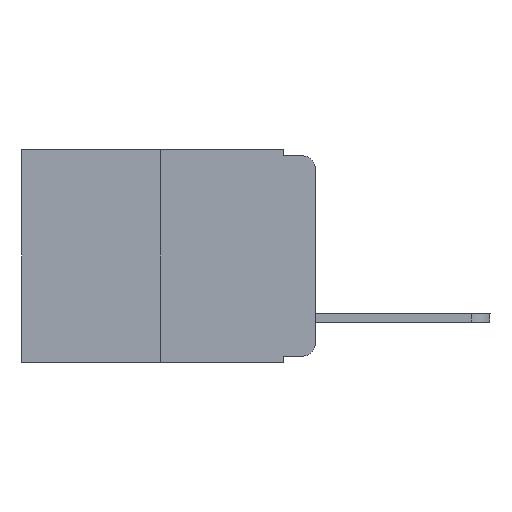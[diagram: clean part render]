
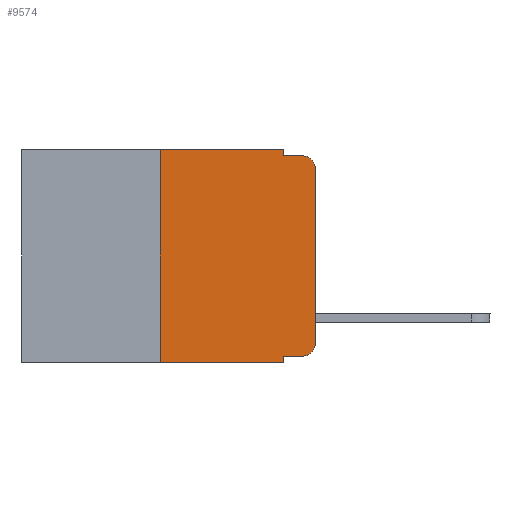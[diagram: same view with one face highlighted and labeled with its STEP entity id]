
A CAD part, left-side view. The second image highlights one B-rep face of the part: STEP entity #9574.
In plain terms, the highlighted planar face has unit normal (-1, 0, 0).
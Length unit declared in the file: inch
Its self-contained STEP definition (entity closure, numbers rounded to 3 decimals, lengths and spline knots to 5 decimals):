
#518 = CARTESIAN_POINT ( 'NONE',  ( 0., 0.02, -0.03 ) ) ;
#831 = DIRECTION ( 'NONE',  ( -1., 0., 0. ) ) ;
#873 = EDGE_LOOP ( 'NONE', ( #3784, #8087, #7034, #19540, #10809, #8668, #8535, #2222, #12883, #15173 ) ) ;
#1061 = LINE ( 'NONE', #19405, #1389 ) ;
#1174 = CARTESIAN_POINT ( 'NONE',  ( 0., 0.02, -0.313 ) ) ;
#1389 = VECTOR ( 'NONE', #11423, 39.37008 ) ;
#1435 = LINE ( 'NONE', #15601, #15882 ) ;
#1588 = CARTESIAN_POINT ( 'NONE',  ( 0., 0.051, 0. ) ) ;
#1994 = LINE ( 'NONE', #3849, #14591 ) ;
#2222 = ORIENTED_EDGE ( 'NONE', *, *, #19116, .F. ) ;
#2387 = EDGE_CURVE ( 'NONE', #11738, #17434, #1435, .T. ) ;
#3282 = CARTESIAN_POINT ( 'NONE',  ( 0., 0., -0.03 ) ) ;
#3784 = ORIENTED_EDGE ( 'NONE', *, *, #24043, .T. ) ;
#3849 = CARTESIAN_POINT ( 'NONE',  ( 0., 0., 0. ) ) ;
#4148 = AXIS2_PLACEMENT_3D ( 'NONE', #518, #22100, #8493 ) ;
#5404 = CARTESIAN_POINT ( 'NONE',  ( 0., 0.051, -0.333 ) ) ;
#6978 = LINE ( 'NONE', #7891, #9766 ) ;
#7034 = ORIENTED_EDGE ( 'NONE', *, *, #2387, .F. ) ;
#7045 = DIRECTION ( 'NONE',  ( 0., 0., 1. ) ) ;
#7232 = EDGE_CURVE ( 'NONE', #15763, #18073, #17824, .T. ) ;
#7244 = CIRCLE ( 'NONE', #4148, 0.02 ) ;
#7891 = CARTESIAN_POINT ( 'NONE',  ( 0., 0.051, 0. ) ) ;
#8087 = ORIENTED_EDGE ( 'NONE', *, *, #24436, .T. ) ;
#8136 = CARTESIAN_POINT ( 'NONE',  ( 0., 0.02, -0.01 ) ) ;
#8482 = CARTESIAN_POINT ( 'NONE',  ( 0., 0.051, -0.333 ) ) ;
#8493 = DIRECTION ( 'NONE',  ( 0., 0., -1. ) ) ;
#8535 = ORIENTED_EDGE ( 'NONE', *, *, #22345, .T. ) ;
#8668 = ORIENTED_EDGE ( 'NONE', *, *, #12371, .F. ) ;
#9007 = VERTEX_POINT ( 'NONE', #13498 ) ;
#9574 = ADVANCED_FACE ( 'NONE', ( #18085 ), #23467, .F. ) ;
#9766 = VECTOR ( 'NONE', #11750, 39.37008 ) ;
#10382 = DIRECTION ( 'NONE',  ( 0., -1., 0. ) ) ;
#10468 = LINE ( 'NONE', #23230, #25074 ) ;
#10804 = DIRECTION ( 'NONE',  ( 0., 0., -1. ) ) ;
#10809 = ORIENTED_EDGE ( 'NONE', *, *, #19938, .F. ) ;
#10907 = CARTESIAN_POINT ( 'NONE',  ( 0., 0.051, -0.01 ) ) ;
#11133 = EDGE_CURVE ( 'NONE', #13557, #11738, #1061, .T. ) ;
#11423 = DIRECTION ( 'NONE',  ( 0., 0., -1. ) ) ;
#11502 = VERTEX_POINT ( 'NONE', #3282 ) ;
#11738 = VERTEX_POINT ( 'NONE', #10907 ) ;
#11750 = DIRECTION ( 'NONE',  ( 0., 0., -1. ) ) ;
#12371 = EDGE_CURVE ( 'NONE', #20728, #12665, #13616, .T. ) ;
#12623 = VECTOR ( 'NONE', #10382, 39.37008 ) ;
#12665 = VERTEX_POINT ( 'NONE', #19398 ) ;
#12883 = ORIENTED_EDGE ( 'NONE', *, *, #7232, .T. ) ;
#13142 = DIRECTION ( 'NONE',  ( 0., 0., -1. ) ) ;
#13294 = VECTOR ( 'NONE', #22021, 39.37008 ) ;
#13498 = CARTESIAN_POINT ( 'NONE',  ( 0., 0., -0.313 ) ) ;
#13557 = VERTEX_POINT ( 'NONE', #1588 ) ;
#13616 = LINE ( 'NONE', #14292, #13294 ) ;
#13661 = CARTESIAN_POINT ( 'NONE',  ( 0., 0.25, -0.343 ) ) ;
#13800 = DIRECTION ( 'NONE',  ( 0., -1., 0. ) ) ;
#14292 = CARTESIAN_POINT ( 'NONE',  ( 0., 0.25, 0. ) ) ;
#14591 = VECTOR ( 'NONE', #7045, 39.37008 ) ;
#15173 = ORIENTED_EDGE ( 'NONE', *, *, #25037, .T. ) ;
#15601 = CARTESIAN_POINT ( 'NONE',  ( 0., 0.051, -0.01 ) ) ;
#15632 = DIRECTION ( 'NONE',  ( 1., 0., 0. ) ) ;
#15763 = VERTEX_POINT ( 'NONE', #5404 ) ;
#15882 = VECTOR ( 'NONE', #13800, 39.37008 ) ;
#16668 = AXIS2_PLACEMENT_3D ( 'NONE', #1174, #831, #10804 ) ;
#16928 = CARTESIAN_POINT ( 'NONE',  ( 0., 0.051, -0.343 ) ) ;
#17381 = LINE ( 'NONE', #24746, #21279 ) ;
#17434 = VERTEX_POINT ( 'NONE', #8136 ) ;
#17824 = LINE ( 'NONE', #8482, #12623 ) ;
#18073 = VERTEX_POINT ( 'NONE', #24046 ) ;
#18085 = FACE_OUTER_BOUND ( 'NONE', #873, .T. ) ;
#19110 = CIRCLE ( 'NONE', #16668, 0.02 ) ;
#19116 = EDGE_CURVE ( 'NONE', #15763, #24598, #6978, .T. ) ;
#19398 = CARTESIAN_POINT ( 'NONE',  ( 0., 0.25, 0. ) ) ;
#19405 = CARTESIAN_POINT ( 'NONE',  ( 0., 0.051, 0. ) ) ;
#19540 = ORIENTED_EDGE ( 'NONE', *, *, #11133, .F. ) ;
#19938 = EDGE_CURVE ( 'NONE', #12665, #13557, #10468, .T. ) ;
#20728 = VERTEX_POINT ( 'NONE', #13661 ) ;
#21279 = VECTOR ( 'NONE', #22449, 39.37008 ) ;
#22021 = DIRECTION ( 'NONE',  ( 0., 0., 1. ) ) ;
#22100 = DIRECTION ( 'NONE',  ( -1., 0., 0. ) ) ;
#22345 = EDGE_CURVE ( 'NONE', #20728, #24598, #17381, .T. ) ;
#22449 = DIRECTION ( 'NONE',  ( 0., -1., 0. ) ) ;
#23230 = CARTESIAN_POINT ( 'NONE',  ( 0., 0.473, 0. ) ) ;
#23406 = DIRECTION ( 'NONE',  ( 0., -1., 0. ) ) ;
#23467 = PLANE ( 'NONE',  #23764 ) ;
#23764 = AXIS2_PLACEMENT_3D ( 'NONE', #24812, #15632, #13142 ) ;
#24043 = EDGE_CURVE ( 'NONE', #9007, #11502, #1994, .T. ) ;
#24046 = CARTESIAN_POINT ( 'NONE',  ( 0., 0.02, -0.333 ) ) ;
#24436 = EDGE_CURVE ( 'NONE', #11502, #17434, #7244, .T. ) ;
#24598 = VERTEX_POINT ( 'NONE', #16928 ) ;
#24746 = CARTESIAN_POINT ( 'NONE',  ( 0., 0.473, -0.343 ) ) ;
#24812 = CARTESIAN_POINT ( 'NONE',  ( 0., 0.473, 0. ) ) ;
#25037 = EDGE_CURVE ( 'NONE', #18073, #9007, #19110, .T. ) ;
#25074 = VECTOR ( 'NONE', #23406, 39.37008 ) ;
